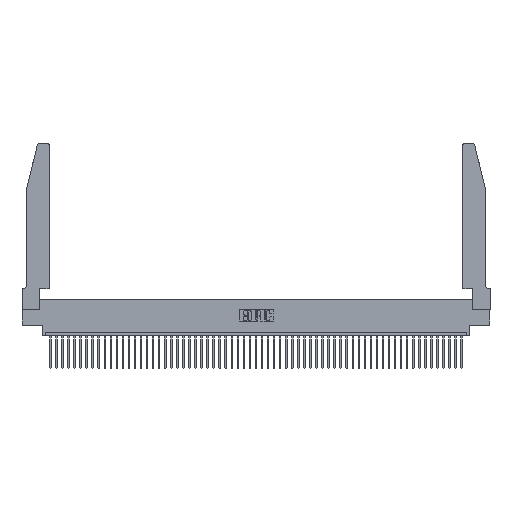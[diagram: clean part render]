
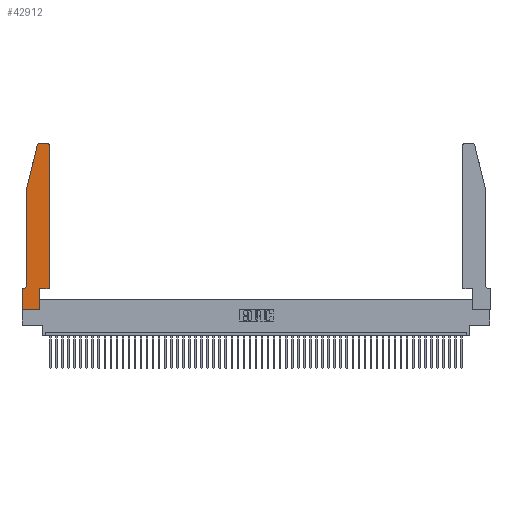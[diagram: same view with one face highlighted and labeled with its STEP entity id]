
A CAD part, top view. The second image highlights one B-rep face of the part: STEP entity #42912.
In plain terms, the highlighted planar face has unit normal (0, 0, 1).
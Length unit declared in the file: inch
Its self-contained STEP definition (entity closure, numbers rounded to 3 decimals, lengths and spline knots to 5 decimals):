
#1812 = DIRECTION ( 'NONE',  ( 0., 0., -1. ) ) ;
#1858 = CARTESIAN_POINT ( 'NONE',  ( 0.25487, 2.72718, 0.37 ) ) ;
#2967 = LINE ( 'NONE', #30170, #45856 ) ;
#3882 = VECTOR ( 'NONE', #34493, 39.37008 ) ;
#4087 = DIRECTION ( 'NONE',  ( 1., 0., 0. ) ) ;
#4385 = EDGE_LOOP ( 'NONE', ( #37983, #21284, #46537, #46425, #12280, #48461, #20798, #9623, #16971, #30870, #34048, #36380 ) ) ;
#5354 = LINE ( 'NONE', #51661, #9169 ) ;
#9169 = VECTOR ( 'NONE', #18409, 39.37008 ) ;
#9379 = LINE ( 'NONE', #51338, #51883 ) ;
#9623 = ORIENTED_EDGE ( 'NONE', *, *, #36844, .T. ) ;
#9907 = DIRECTION ( 'NONE',  ( -1., 0., 0. ) ) ;
#10131 = CARTESIAN_POINT ( 'NONE',  ( 0.2865, 0., 0.37 ) ) ;
#10185 = EDGE_CURVE ( 'NONE', #49537, #44672, #16057, .T. ) ;
#10423 = EDGE_CURVE ( 'NONE', #31787, #18648, #42330, .T. ) ;
#12280 = ORIENTED_EDGE ( 'NONE', *, *, #10423, .T. ) ;
#13205 = VERTEX_POINT ( 'NONE', #19628 ) ;
#13964 = CARTESIAN_POINT ( 'NONE',  ( 0.2865, 0.35, 0.37 ) ) ;
#13983 = CARTESIAN_POINT ( 'NONE',  ( 0.2605, 2.75, 0.37 ) ) ;
#14280 = VERTEX_POINT ( 'NONE', #22764 ) ;
#15204 = CARTESIAN_POINT ( 'NONE',  ( 0.4205, 2.75, 0.37 ) ) ;
#16057 = LINE ( 'NONE', #13983, #3882 ) ;
#16251 = DIRECTION ( 'NONE',  ( 0., 0., 1. ) ) ;
#16971 = ORIENTED_EDGE ( 'NONE', *, *, #22609, .T. ) ;
#17469 = LINE ( 'NONE', #25850, #40714 ) ;
#17565 = DIRECTION ( 'NONE',  ( -1., 0., 0. ) ) ;
#17711 = DIRECTION ( 'NONE',  ( 1., 0., 0. ) ) ;
#17835 = VERTEX_POINT ( 'NONE', #35727 ) ;
#18124 = DIRECTION ( 'NONE',  ( 0., 1., 0. ) ) ;
#18409 = DIRECTION ( 'NONE',  ( 1., 0., 0. ) ) ;
#18648 = VERTEX_POINT ( 'NONE', #21982 ) ;
#19322 = CARTESIAN_POINT ( 'NONE',  ( 0., 0., 0.37 ) ) ;
#19628 = CARTESIAN_POINT ( 'NONE',  ( 0., 0., 0.37 ) ) ;
#20798 = ORIENTED_EDGE ( 'NONE', *, *, #50774, .T. ) ;
#20839 = PLANE ( 'NONE',  #46755 ) ;
#20986 = CARTESIAN_POINT ( 'NONE',  ( 0.4505, 2.72, 0.37 ) ) ;
#21284 = ORIENTED_EDGE ( 'NONE', *, *, #53033, .T. ) ;
#21827 = CARTESIAN_POINT ( 'NONE',  ( 0.4205, 2.72, 0.37 ) ) ;
#21982 = CARTESIAN_POINT ( 'NONE',  ( 0.0055, 0.35, 0.37 ) ) ;
#22609 = EDGE_CURVE ( 'NONE', #52170, #35411, #17469, .T. ) ;
#22764 = CARTESIAN_POINT ( 'NONE',  ( 0., 0.35, 0.37 ) ) ;
#25799 = DIRECTION ( 'NONE',  ( 0., 0., 1. ) ) ;
#25850 = CARTESIAN_POINT ( 'NONE',  ( 0.2865, 0.35, 0.37 ) ) ;
#26185 = AXIS2_PLACEMENT_3D ( 'NONE', #26246, #1812, #9907 ) ;
#26246 = CARTESIAN_POINT ( 'NONE',  ( 0.0055, 0.42, 0.37 ) ) ;
#26721 = EDGE_CURVE ( 'NONE', #30562, #17835, #9379, .T. ) ;
#27805 = CARTESIAN_POINT ( 'NONE',  ( 0.4505, 0.35, 0.37 ) ) ;
#28842 = CARTESIAN_POINT ( 'NONE',  ( 0., 0.35, 0.37 ) ) ;
#29824 = DIRECTION ( 'NONE',  ( 0., -1., 0. ) ) ;
#30170 = CARTESIAN_POINT ( 'NONE',  ( 0., 0., 0.37 ) ) ;
#30218 = DIRECTION ( 'NONE',  ( 0., -1., 0. ) ) ;
#30562 = VERTEX_POINT ( 'NONE', #1858 ) ;
#30574 = LINE ( 'NONE', #27805, #36437 ) ;
#30870 = ORIENTED_EDGE ( 'NONE', *, *, #43884, .T. ) ;
#31787 = VERTEX_POINT ( 'NONE', #40565 ) ;
#32255 = DIRECTION ( 'NONE',  ( 1., 0., 0. ) ) ;
#32422 = VECTOR ( 'NONE', #17565, 39.37008 ) ;
#32960 = DIRECTION ( 'NONE',  ( 1., 0., 0. ) ) ;
#33748 = FACE_OUTER_BOUND ( 'NONE', #4385, .T. ) ;
#33903 = VECTOR ( 'NONE', #32960, 39.37008 ) ;
#33959 = CIRCLE ( 'NONE', #41624, 0.03 ) ;
#34048 = ORIENTED_EDGE ( 'NONE', *, *, #38018, .T. ) ;
#34493 = DIRECTION ( 'NONE',  ( -1., 0., 0. ) ) ;
#34963 = LINE ( 'NONE', #49168, #32422 ) ;
#35326 = CARTESIAN_POINT ( 'NONE',  ( 0.284, 2.75, 0.37 ) ) ;
#35411 = VERTEX_POINT ( 'NONE', #13964 ) ;
#35727 = CARTESIAN_POINT ( 'NONE',  ( 0.0755, 2., 0.37 ) ) ;
#36380 = ORIENTED_EDGE ( 'NONE', *, *, #51358, .T. ) ;
#36437 = VECTOR ( 'NONE', #48698, 39.37008 ) ;
#36844 = EDGE_CURVE ( 'NONE', #13205, #52170, #44889, .T. ) ;
#37395 = EDGE_CURVE ( 'NONE', #17835, #31787, #40330, .T. ) ;
#37755 = AXIS2_PLACEMENT_3D ( 'NONE', #21827, #25799, #17711 ) ;
#37983 = ORIENTED_EDGE ( 'NONE', *, *, #10185, .T. ) ;
#38018 = EDGE_CURVE ( 'NONE', #47492, #45874, #30574, .T. ) ;
#39008 = DIRECTION ( 'NONE',  ( -0.239, -0.971, 0. ) ) ;
#39774 = CARTESIAN_POINT ( 'NONE',  ( 0.284, 2.72, 0.37 ) ) ;
#40330 = LINE ( 'NONE', #51389, #44837 ) ;
#40565 = CARTESIAN_POINT ( 'NONE',  ( 0.0755, 0.42, 0.37 ) ) ;
#40714 = VECTOR ( 'NONE', #18124, 39.37008 ) ;
#41624 = AXIS2_PLACEMENT_3D ( 'NONE', #39774, #47980, #32255 ) ;
#42330 = CIRCLE ( 'NONE', #26185, 0.07 ) ;
#42912 = ADVANCED_FACE ( 'NONE', ( #33748 ), #20839, .T. ) ;
#43699 = CARTESIAN_POINT ( 'NONE',  ( 0.4505, 0.35, 0.37 ) ) ;
#43884 = EDGE_CURVE ( 'NONE', #35411, #47492, #5354, .T. ) ;
#44672 = VERTEX_POINT ( 'NONE', #35326 ) ;
#44833 = EDGE_CURVE ( 'NONE', #18648, #14280, #34963, .T. ) ;
#44837 = VECTOR ( 'NONE', #30218, 39.37008 ) ;
#44889 = LINE ( 'NONE', #19322, #33903 ) ;
#45229 = CIRCLE ( 'NONE', #37755, 0.03 ) ;
#45856 = VECTOR ( 'NONE', #29824, 39.37008 ) ;
#45874 = VERTEX_POINT ( 'NONE', #20986 ) ;
#46425 = ORIENTED_EDGE ( 'NONE', *, *, #37395, .T. ) ;
#46537 = ORIENTED_EDGE ( 'NONE', *, *, #26721, .T. ) ;
#46755 = AXIS2_PLACEMENT_3D ( 'NONE', #28842, #16251, #4087 ) ;
#47492 = VERTEX_POINT ( 'NONE', #43699 ) ;
#47980 = DIRECTION ( 'NONE',  ( 0., 0., 1. ) ) ;
#48461 = ORIENTED_EDGE ( 'NONE', *, *, #44833, .T. ) ;
#48698 = DIRECTION ( 'NONE',  ( 0., 1., 0. ) ) ;
#49168 = CARTESIAN_POINT ( 'NONE',  ( 0.0755, 0.35, 0.37 ) ) ;
#49537 = VERTEX_POINT ( 'NONE', #15204 ) ;
#50774 = EDGE_CURVE ( 'NONE', #14280, #13205, #2967, .T. ) ;
#51338 = CARTESIAN_POINT ( 'NONE',  ( 0.0755, 2., 0.37 ) ) ;
#51358 = EDGE_CURVE ( 'NONE', #45874, #49537, #45229, .T. ) ;
#51389 = CARTESIAN_POINT ( 'NONE',  ( 0.0755, 2., 0.37 ) ) ;
#51661 = CARTESIAN_POINT ( 'NONE',  ( 0.4505, 0.35, 0.37 ) ) ;
#51883 = VECTOR ( 'NONE', #39008, 39.37008 ) ;
#52170 = VERTEX_POINT ( 'NONE', #10131 ) ;
#53033 = EDGE_CURVE ( 'NONE', #44672, #30562, #33959, .T. ) ;
